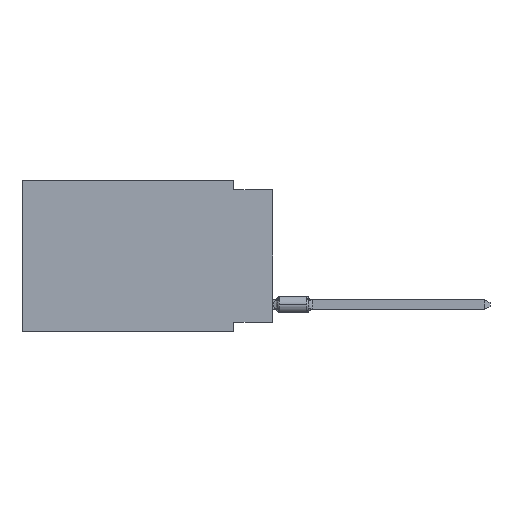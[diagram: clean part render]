
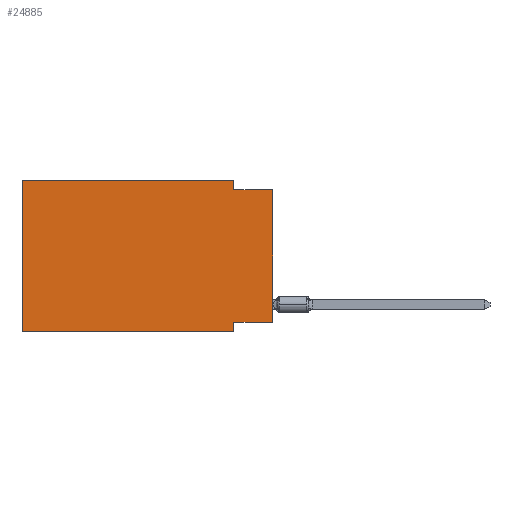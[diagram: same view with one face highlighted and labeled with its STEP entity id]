
A CAD part, left-side view. The second image highlights one B-rep face of the part: STEP entity #24885.
In plain terms, the highlighted planar face has unit normal (-1, 0, 0).
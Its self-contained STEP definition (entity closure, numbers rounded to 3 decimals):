
#296 = LINE ( 'NONE', #8911, #25994 ) ;
#547 = CARTESIAN_POINT ( 'NONE',  ( 0., 2.54, -0.635 ) ) ;
#888 = LINE ( 'NONE', #18220, #6572 ) ;
#961 = EDGE_CURVE ( 'NONE', #8138, #24951, #6992, .T. ) ;
#1067 = VECTOR ( 'NONE', #12276, 1000. ) ;
#3396 = EDGE_CURVE ( 'NONE', #24146, #19088, #888, .T. ) ;
#3453 = ORIENTED_EDGE ( 'NONE', *, *, #20159, .T. ) ;
#3660 = CARTESIAN_POINT ( 'NONE',  ( 0., 0., -9.271 ) ) ;
#3803 = ORIENTED_EDGE ( 'NONE', *, *, #961, .F. ) ;
#3967 = FACE_OUTER_BOUND ( 'NONE', #11668, .T. ) ;
#4154 = LINE ( 'NONE', #12763, #7539 ) ;
#4739 = ORIENTED_EDGE ( 'NONE', *, *, #26170, .F. ) ;
#5015 = CARTESIAN_POINT ( 'NONE',  ( 0., 16.383, 0. ) ) ;
#6008 = EDGE_CURVE ( 'NONE', #24951, #8837, #4154, .T. ) ;
#6382 = EDGE_CURVE ( 'NONE', #23764, #19088, #296, .T. ) ;
#6572 = VECTOR ( 'NONE', #16256, 1000. ) ;
#6992 = LINE ( 'NONE', #13593, #16994 ) ;
#7539 = VECTOR ( 'NONE', #21359, 1000. ) ;
#7833 = VERTEX_POINT ( 'NONE', #25173 ) ;
#8077 = DIRECTION ( 'NONE',  ( 0., 0., 1. ) ) ;
#8138 = VERTEX_POINT ( 'NONE', #5015 ) ;
#8574 = ORIENTED_EDGE ( 'NONE', *, *, #3396, .T. ) ;
#8634 = CARTESIAN_POINT ( 'NONE',  ( 0., 16.383, 0. ) ) ;
#8837 = VERTEX_POINT ( 'NONE', #547 ) ;
#8911 = CARTESIAN_POINT ( 'NONE',  ( 0., 2.54, -9.906 ) ) ;
#9818 = EDGE_CURVE ( 'NONE', #24146, #8138, #10761, .T. ) ;
#10448 = CARTESIAN_POINT ( 'NONE',  ( 0., 16.383, 0. ) ) ;
#10761 = LINE ( 'NONE', #8634, #19081 ) ;
#10790 = VERTEX_POINT ( 'NONE', #25579 ) ;
#10930 = ORIENTED_EDGE ( 'NONE', *, *, #6382, .F. ) ;
#11303 = CARTESIAN_POINT ( 'NONE',  ( 0., 2.54, 0. ) ) ;
#11668 = EDGE_LOOP ( 'NONE', ( #3453, #13156, #20769, #3803, #15124, #8574, #10930, #4739 ) ) ;
#12276 = DIRECTION ( 'NONE',  ( 0., 1., 0. ) ) ;
#12329 = DIRECTION ( 'NONE',  ( 0., 0., 1. ) ) ;
#12572 = PLANE ( 'NONE',  #13230 ) ;
#12763 = CARTESIAN_POINT ( 'NONE',  ( 0., 2.54, 0. ) ) ;
#13156 = ORIENTED_EDGE ( 'NONE', *, *, #24529, .F. ) ;
#13230 = AXIS2_PLACEMENT_3D ( 'NONE', #10448, #26633, #15673 ) ;
#13593 = CARTESIAN_POINT ( 'NONE',  ( 0., 16.383, 0. ) ) ;
#14386 = LINE ( 'NONE', #3660, #1067 ) ;
#15006 = CARTESIAN_POINT ( 'NONE',  ( 0., 2.54, -9.906 ) ) ;
#15124 = ORIENTED_EDGE ( 'NONE', *, *, #9818, .F. ) ;
#15483 = CARTESIAN_POINT ( 'NONE',  ( 0., 16.383, -9.906 ) ) ;
#15575 = DIRECTION ( 'NONE',  ( 0., -1., 0. ) ) ;
#15673 = DIRECTION ( 'NONE',  ( 0., 0., -1. ) ) ;
#15944 = CARTESIAN_POINT ( 'NONE',  ( 0., 2.54, -9.271 ) ) ;
#16256 = DIRECTION ( 'NONE',  ( 0., -1., 0. ) ) ;
#16417 = LINE ( 'NONE', #25017, #16788 ) ;
#16788 = VECTOR ( 'NONE', #12329, 1000. ) ;
#16994 = VECTOR ( 'NONE', #15575, 1000. ) ;
#17492 = DIRECTION ( 'NONE',  ( 0., 0., -1. ) ) ;
#18220 = CARTESIAN_POINT ( 'NONE',  ( 0., 16.383, -9.906 ) ) ;
#19060 = CARTESIAN_POINT ( 'NONE',  ( 0., 0., -0.635 ) ) ;
#19081 = VECTOR ( 'NONE', #8077, 1000. ) ;
#19088 = VERTEX_POINT ( 'NONE', #15006 ) ;
#19344 = DIRECTION ( 'NONE',  ( 0., -1., 0. ) ) ;
#20159 = EDGE_CURVE ( 'NONE', #7833, #10790, #16417, .T. ) ;
#20769 = ORIENTED_EDGE ( 'NONE', *, *, #6008, .F. ) ;
#21359 = DIRECTION ( 'NONE',  ( 0., 0., -1. ) ) ;
#21902 = LINE ( 'NONE', #19060, #27570 ) ;
#23764 = VERTEX_POINT ( 'NONE', #15944 ) ;
#24146 = VERTEX_POINT ( 'NONE', #15483 ) ;
#24529 = EDGE_CURVE ( 'NONE', #8837, #10790, #21902, .T. ) ;
#24885 = ADVANCED_FACE ( 'NONE', ( #3967 ), #12572, .F. ) ;
#24951 = VERTEX_POINT ( 'NONE', #11303 ) ;
#25017 = CARTESIAN_POINT ( 'NONE',  ( 0., 0., 0. ) ) ;
#25173 = CARTESIAN_POINT ( 'NONE',  ( 0., 0., -9.271 ) ) ;
#25579 = CARTESIAN_POINT ( 'NONE',  ( 0., 0., -0.635 ) ) ;
#25994 = VECTOR ( 'NONE', #17492, 1000. ) ;
#26170 = EDGE_CURVE ( 'NONE', #7833, #23764, #14386, .T. ) ;
#26633 = DIRECTION ( 'NONE',  ( 1., 0., 0. ) ) ;
#27570 = VECTOR ( 'NONE', #19344, 1000. ) ;
